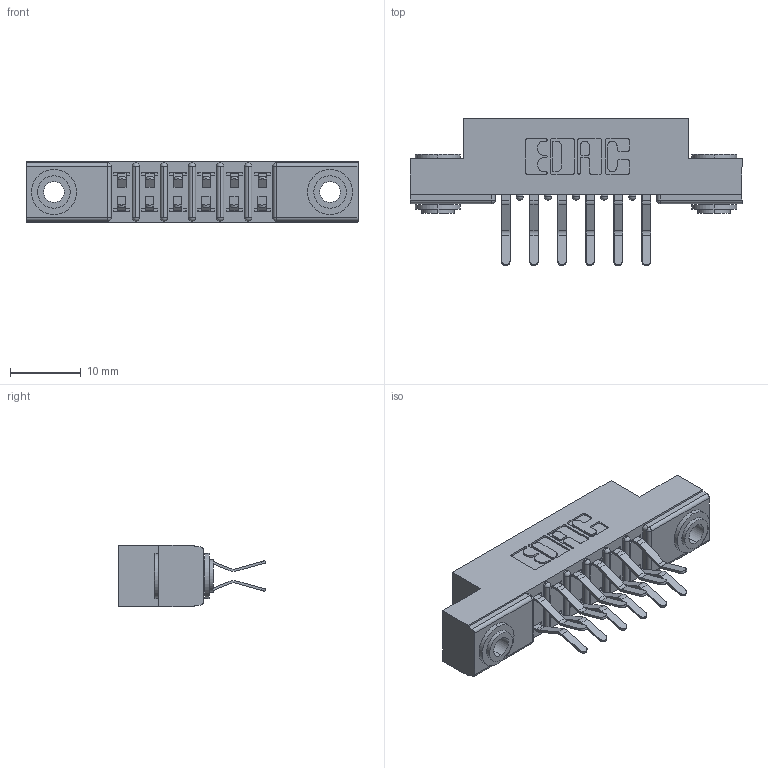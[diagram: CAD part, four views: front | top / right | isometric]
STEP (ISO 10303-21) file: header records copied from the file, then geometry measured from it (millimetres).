
FILE_DESCRIPTION (( 'STEP AP203' ), '1' );
FILE_NAME ('307-012-460-203.STEP', '2020-09-28T15:15:08', ( '' ), ( '' ), 'SwSTEP 2.0', 'SolidWorks 2020', '' );
FILE_SCHEMA (( 'CONFIG_CONTROL_DESIGN' ));
Length unit declared in the file: inch
Products named in the file (4): 345-250-002_345-250-002-102; 307-012-460-203; 307-290-001_560; 307 Part_.156 Dia Mounting Holes
Assembly tree (15 placements, depth 2):
  307-012-460-203
    307 Part_.156 Dia Mounting Holes
    307-290-001_560  x12
    345-250-002_345-250-002-102  x2
Bounding box: 46.79 x 20.73 x 8.71 mm (x, y, z)
Volume: 3078.4 mm3; surface area: 4941 mm2
Topology: 15 solids, 15 shells, 777 faces, 2139 edges, 1386 vertices
Faces by surface type: plane 490, cylinder 265, sphere 14, cone 8
Entity records: 10943 total; most frequent: CARTESIAN_POINT 1783, DIRECTION 1777, ORIENTED_EDGE 1754, EDGE_CURVE 877, LINE 649, VECTOR 649, VERTEX_POINT 570, AXIS2_PLACEMENT_3D 564
